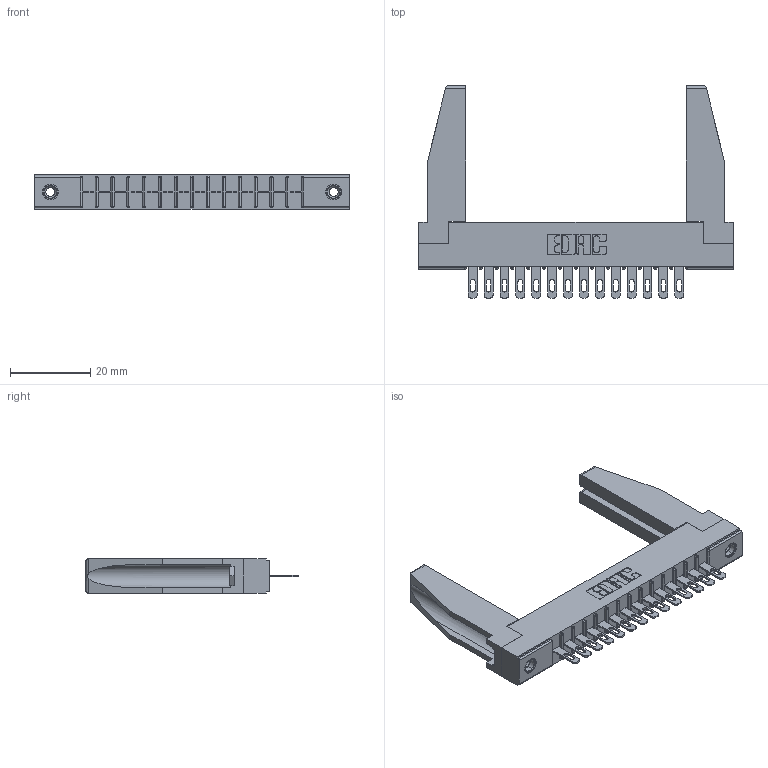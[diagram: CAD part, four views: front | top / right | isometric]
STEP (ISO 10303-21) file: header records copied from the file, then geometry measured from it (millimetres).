
FILE_DESCRIPTION (( 'STEP AP203' ), '1' );
FILE_NAME ('356-014-500-178.STEP', '2018-08-01T19:03:50', ( '' ), ( '' ), 'SwSTEP 2.0', 'SolidWorks 2016', '' );
FILE_SCHEMA (( 'CONFIG_CONTROL_DESIGN' ));
Length unit declared in the file: inch
Products named in the file (5): 306 Part_.156 Dia; 306-290-001_100; 345-250-001_345-250-001-102; 307-220-078; 356-014-500-178
Assembly tree (19 placements, depth 2):
  356-014-500-178
    306 Part_.156 Dia
    306-290-001_100  x14
    345-250-001_345-250-001-102  x2
    307-220-078  x2
Bounding box: 78.49 x 52.91 x 8.71 mm (x, y, z)
Volume: 9366.9 mm3; surface area: 11753.9 mm2
Topology: 19 solids, 19 shells, 1310 faces, 3656 edges, 2352 vertices
Faces by surface type: plane 852, cylinder 386, sphere 56, cone 12, torus 4
Entity records: 19286 total; most frequent: CARTESIAN_POINT 3235, ORIENTED_EDGE 3162, DIRECTION 3145, EDGE_CURVE 1581, VECTOR 1221, LINE 1221, VERTEX_POINT 1010, AXIS2_PLACEMENT_3D 962
